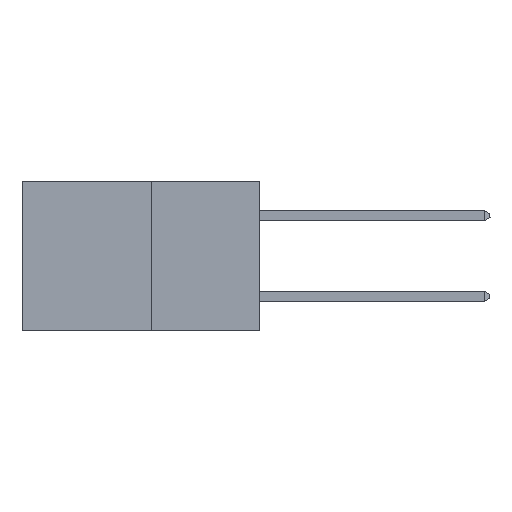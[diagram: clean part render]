
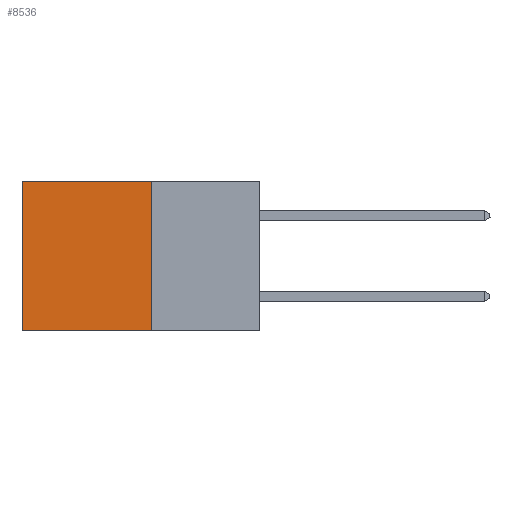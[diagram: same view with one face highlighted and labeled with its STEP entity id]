
A CAD part, left-side view. The second image highlights one B-rep face of the part: STEP entity #8536.
In plain terms, the highlighted planar face has unit normal (-1, 0, 0).
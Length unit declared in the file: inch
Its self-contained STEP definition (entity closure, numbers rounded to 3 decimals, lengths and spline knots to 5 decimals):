
#187 = ORIENTED_EDGE ( 'NONE', *, *, #1764, .F. ) ;
#799 = CARTESIAN_POINT ( 'NONE',  ( 0.277, 0.27, -0.37 ) ) ;
#1356 = DIRECTION ( 'NONE',  ( 0., 0., -1. ) ) ;
#1508 = VERTEX_POINT ( 'NONE', #12808 ) ;
#1591 = FACE_OUTER_BOUND ( 'NONE', #2592, .T. ) ;
#1717 = EDGE_CURVE ( 'NONE', #4025, #2488, #7188, .T. ) ;
#1764 = EDGE_CURVE ( 'NONE', #8476, #1508, #9985, .T. ) ;
#1808 = CARTESIAN_POINT ( 'NONE',  ( 0.277, 0.59, 0. ) ) ;
#1862 = EDGE_CURVE ( 'NONE', #8476, #4025, #5290, .T. ) ;
#2488 = VERTEX_POINT ( 'NONE', #7854 ) ;
#2592 = EDGE_LOOP ( 'NONE', ( #9588, #13449, #187, #12633 ) ) ;
#2606 = CARTESIAN_POINT ( 'NONE',  ( 0.277, 0.59, -0.37 ) ) ;
#2733 = DIRECTION ( 'NONE',  ( 0., 0., -1. ) ) ;
#3148 = VECTOR ( 'NONE', #3722, 39.37008 ) ;
#3722 = DIRECTION ( 'NONE',  ( 0., 0., -1. ) ) ;
#3946 = CARTESIAN_POINT ( 'NONE',  ( 0.277, 0.27, -0.37 ) ) ;
#4025 = VERTEX_POINT ( 'NONE', #1808 ) ;
#4340 = AXIS2_PLACEMENT_3D ( 'NONE', #7568, #8724, #1356 ) ;
#4995 = CARTESIAN_POINT ( 'NONE',  ( 0.277, 0.27, 0. ) ) ;
#5290 = LINE ( 'NONE', #11359, #8128 ) ;
#7102 = DIRECTION ( 'NONE',  ( 0., 1., 0. ) ) ;
#7188 = LINE ( 'NONE', #2606, #13155 ) ;
#7568 = CARTESIAN_POINT ( 'NONE',  ( 0.277, 0.27, -0.37 ) ) ;
#7854 = CARTESIAN_POINT ( 'NONE',  ( 0.277, 0.59, -0.37 ) ) ;
#8128 = VECTOR ( 'NONE', #11810, 39.37008 ) ;
#8476 = VERTEX_POINT ( 'NONE', #4995 ) ;
#8532 = VECTOR ( 'NONE', #7102, 39.37008 ) ;
#8536 = ADVANCED_FACE ( 'NONE', ( #1591 ), #14676, .F. ) ;
#8724 = DIRECTION ( 'NONE',  ( 1., 0., 0. ) ) ;
#9588 = ORIENTED_EDGE ( 'NONE', *, *, #1717, .T. ) ;
#9985 = LINE ( 'NONE', #3946, #3148 ) ;
#11359 = CARTESIAN_POINT ( 'NONE',  ( 0.277, 0.27, 0. ) ) ;
#11737 = LINE ( 'NONE', #799, #8532 ) ;
#11810 = DIRECTION ( 'NONE',  ( 0., 1., 0. ) ) ;
#11924 = EDGE_CURVE ( 'NONE', #1508, #2488, #11737, .T. ) ;
#12633 = ORIENTED_EDGE ( 'NONE', *, *, #1862, .T. ) ;
#12808 = CARTESIAN_POINT ( 'NONE',  ( 0.277, 0.27, -0.37 ) ) ;
#13155 = VECTOR ( 'NONE', #2733, 39.37008 ) ;
#13449 = ORIENTED_EDGE ( 'NONE', *, *, #11924, .F. ) ;
#14676 = PLANE ( 'NONE',  #4340 ) ;
